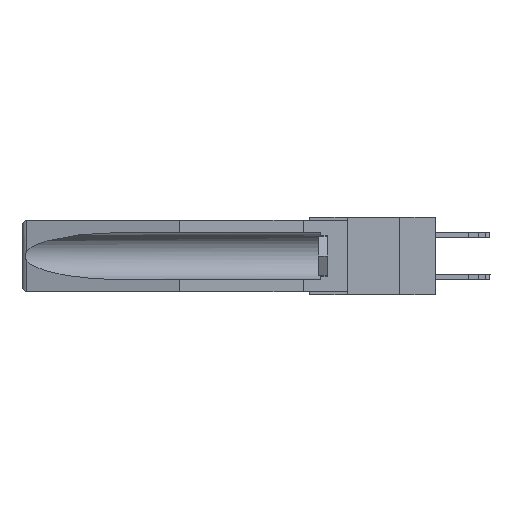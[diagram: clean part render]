
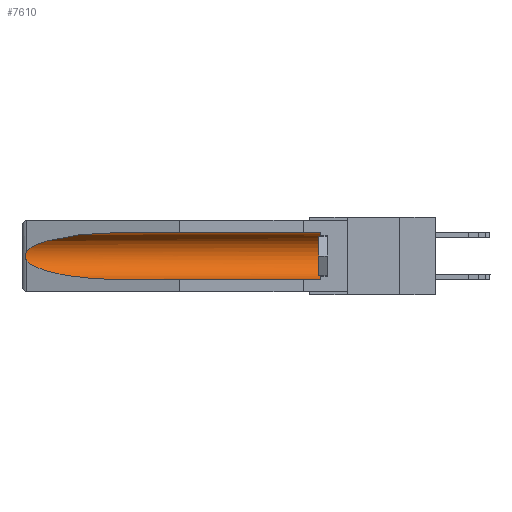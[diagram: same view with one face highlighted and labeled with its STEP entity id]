
A CAD part, left-side view. The second image highlights one B-rep face of the part: STEP entity #7610.
In plain terms, the highlighted cylindrical face has radius 2.857 mm (diameter 5.715 mm), a partial arc.
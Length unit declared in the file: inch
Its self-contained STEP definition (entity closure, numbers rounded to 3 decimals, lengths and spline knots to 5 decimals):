
#242 = CARTESIAN_POINT ( 'NONE',  ( 0.25451, 1.48313, -0.09465 ) ) ;
#259 = VERTEX_POINT ( 'NONE', #16874 ) ;
#636 = ORIENTED_EDGE ( 'NONE', *, *, #17606, .T. ) ;
#1351 = EDGE_LOOP ( 'NONE', ( #13171, #9203, #16465, #19913, #636, #8692 ) ) ;
#1501 = VECTOR ( 'NONE', #2308, 39.37008 ) ;
#1729 = CARTESIAN_POINT ( 'NONE',  ( 0.2673, 1.5327, -0.16383 ) ) ;
#2183 = VERTEX_POINT ( 'NONE', #19014 ) ;
#2308 = DIRECTION ( 'NONE',  ( 0., 1., 0. ) ) ;
#2413 = DIRECTION ( 'NONE',  ( 0., 0., 1. ) ) ;
#2492 = DIRECTION ( 'NONE',  ( 0., 1., 0. ) ) ;
#2912 = EDGE_CURVE ( 'NONE', #5879, #17378, #12004, .T. ) ;
#3170 =( BOUNDED_CURVE ( )  B_SPLINE_CURVE ( 3, ( #5510, #18207, #242, #13255 ),
 .UNSPECIFIED., .F., .F. ) 
 B_SPLINE_CURVE_WITH_KNOTS ( ( 4, 4 ),
 ( 4.71239, 6.08839 ),
 .UNSPECIFIED. ) 
 CURVE ( )  GEOMETRIC_REPRESENTATION_ITEM ( )  RATIONAL_B_SPLINE_CURVE ( ( 1., 0.848, 0.848, 1. ) ) 
 REPRESENTATION_ITEM ( '' )  );
#3363 = VERTEX_POINT ( 'NONE', #12216 ) ;
#3366 = CARTESIAN_POINT ( 'NONE',  ( 0.2675, 1.53308, -0.17534 ) ) ;
#3508 = LINE ( 'NONE', #20313, #22708 ) ;
#4063 = CARTESIAN_POINT ( 'NONE',  ( 0.155, 1.07973, -0.284 ) ) ;
#4111 = CARTESIAN_POINT ( 'NONE',  ( 0.155, -0.30754, -0.284 ) ) ;
#4200 = AXIS2_PLACEMENT_3D ( 'NONE', #22655, #22563, #18745 ) ;
#4344 = CARTESIAN_POINT ( 'NONE',  ( 0.155, 1.07973, -0.059 ) ) ;
#4540 = EDGE_CURVE ( 'NONE', #8351, #2183, #3170, .T. ) ;
#4685 = EDGE_CURVE ( 'NONE', #2183, #3363, #10012, .T. ) ;
#5510 = CARTESIAN_POINT ( 'NONE',  ( 0.155, 1.07973, -0.059 ) ) ;
#5879 = VERTEX_POINT ( 'NONE', #17834 ) ;
#7610 = ADVANCED_FACE ( 'NONE', ( #19064 ), #16478, .F. ) ;
#8351 = VERTEX_POINT ( 'NONE', #4344 ) ;
#8692 = ORIENTED_EDGE ( 'NONE', *, *, #23924, .T. ) ;
#8962 = CARTESIAN_POINT ( 'NONE',  ( 0.26597, 1.5296, -0.19026 ) ) ;
#9203 = ORIENTED_EDGE ( 'NONE', *, *, #4685, .T. ) ;
#10012 = B_SPLINE_CURVE_WITH_KNOTS ( 'NONE', 3,
 ( #22216, #14512, #23871, #1729, #11083, #3366, #18230, #20100, #8962, #14591 ),
 .UNSPECIFIED., .F., .F.,
 ( 4, 2, 2, 2, 4 ),
 ( 0., 0.00029, 0.00058, 0.00087, 0.00117 ),
 .UNSPECIFIED. ) ;
#10620 = CARTESIAN_POINT ( 'NONE',  ( 0.155, 1.07973, -0.284 ) ) ;
#11083 = CARTESIAN_POINT ( 'NONE',  ( 0.2675, 1.53308, -0.16763 ) ) ;
#12004 = LINE ( 'NONE', #4111, #1501 ) ;
#12216 = CARTESIAN_POINT ( 'NONE',  ( 0.26537, 1.52718, -0.19328 ) ) ;
#13171 = ORIENTED_EDGE ( 'NONE', *, *, #4540, .T. ) ;
#13255 = CARTESIAN_POINT ( 'NONE',  ( 0.26537, 1.52718, -0.14972 ) ) ;
#13562 = CARTESIAN_POINT ( 'NONE',  ( 0.155, -0.30754, -0.1715 ) ) ;
#14512 = CARTESIAN_POINT ( 'NONE',  ( 0.26597, 1.52961, -0.15275 ) ) ;
#14591 = CARTESIAN_POINT ( 'NONE',  ( 0.26537, 1.52718, -0.19328 ) ) ;
#14805 = DIRECTION ( 'NONE',  ( 0., 1., 0. ) ) ;
#15034 = CARTESIAN_POINT ( 'NONE',  ( 0.25451, 1.48313, -0.24835 ) ) ;
#15209 = CARTESIAN_POINT ( 'NONE',  ( 0.21114, 1.30732, -0.284 ) ) ;
#16465 = ORIENTED_EDGE ( 'NONE', *, *, #17148, .T. ) ;
#16478 = CYLINDRICAL_SURFACE ( 'NONE', #20704, 0.1125 ) ;
#16874 = CARTESIAN_POINT ( 'NONE',  ( 0.155, 0.126, -0.059 ) ) ;
#17148 = EDGE_CURVE ( 'NONE', #3363, #17378, #19402, .T. ) ;
#17378 = VERTEX_POINT ( 'NONE', #10620 ) ;
#17606 = EDGE_CURVE ( 'NONE', #5879, #259, #21190, .T. ) ;
#17834 = CARTESIAN_POINT ( 'NONE',  ( 0.155, 0.126, -0.284 ) ) ;
#18207 = CARTESIAN_POINT ( 'NONE',  ( 0.21114, 1.30732, -0.059 ) ) ;
#18230 = CARTESIAN_POINT ( 'NONE',  ( 0.2673, 1.53269, -0.17917 ) ) ;
#18745 = DIRECTION ( 'NONE',  ( 0., 0., 1. ) ) ;
#19014 = CARTESIAN_POINT ( 'NONE',  ( 0.26537, 1.52718, -0.14972 ) ) ;
#19064 = FACE_OUTER_BOUND ( 'NONE', #1351, .T. ) ;
#19402 =( BOUNDED_CURVE ( )  B_SPLINE_CURVE ( 3, ( #22679, #15034, #15209, #4063 ),
 .UNSPECIFIED., .F., .F. ) 
 B_SPLINE_CURVE_WITH_KNOTS ( ( 4, 4 ),
 ( 0.1948, 1.5708 ),
 .UNSPECIFIED. ) 
 CURVE ( )  GEOMETRIC_REPRESENTATION_ITEM ( )  RATIONAL_B_SPLINE_CURVE ( ( 1., 0.848, 0.848, 1. ) ) 
 REPRESENTATION_ITEM ( '' )  );
#19913 = ORIENTED_EDGE ( 'NONE', *, *, #2912, .F. ) ;
#20100 = CARTESIAN_POINT ( 'NONE',  ( 0.26655, 1.53094, -0.18657 ) ) ;
#20313 = CARTESIAN_POINT ( 'NONE',  ( 0.155, -0.30754, -0.059 ) ) ;
#20704 = AXIS2_PLACEMENT_3D ( 'NONE', #13562, #2492, #2413 ) ;
#21190 = CIRCLE ( 'NONE', #4200, 0.1125 ) ;
#22216 = CARTESIAN_POINT ( 'NONE',  ( 0.26537, 1.52718, -0.14972 ) ) ;
#22563 = DIRECTION ( 'NONE',  ( 0., -1., 0. ) ) ;
#22655 = CARTESIAN_POINT ( 'NONE',  ( 0.155, 0.126, -0.1715 ) ) ;
#22679 = CARTESIAN_POINT ( 'NONE',  ( 0.26537, 1.52718, -0.19328 ) ) ;
#22708 = VECTOR ( 'NONE', #14805, 39.37008 ) ;
#23871 = CARTESIAN_POINT ( 'NONE',  ( 0.26654, 1.53092, -0.15636 ) ) ;
#23924 = EDGE_CURVE ( 'NONE', #259, #8351, #3508, .T. ) ;
